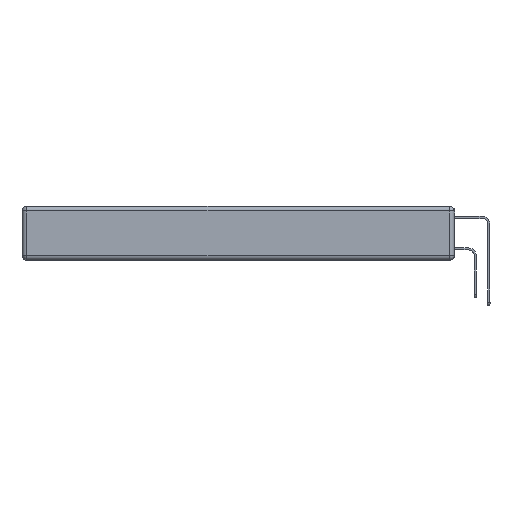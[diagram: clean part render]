
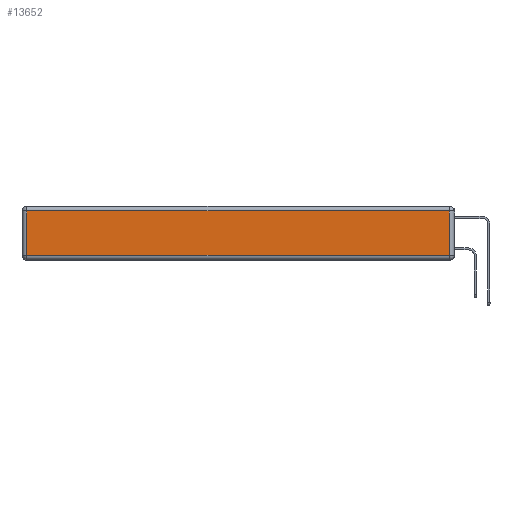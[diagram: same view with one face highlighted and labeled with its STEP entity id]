
A CAD part, left-side view. The second image highlights one B-rep face of the part: STEP entity #13652.
In plain terms, the highlighted planar face has unit normal (-1, 0, 0).
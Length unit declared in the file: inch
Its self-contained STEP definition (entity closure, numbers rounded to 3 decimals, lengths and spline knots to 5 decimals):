
#912 = CARTESIAN_POINT ( 'NONE',  ( 0., 0.03, -0.313 ) ) ;
#995 = DIRECTION ( 'NONE',  ( 0., 0., 1. ) ) ;
#1275 = LINE ( 'NONE', #16826, #14000 ) ;
#2342 = DIRECTION ( 'NONE',  ( 0., 0., 1. ) ) ;
#2383 = VERTEX_POINT ( 'NONE', #912 ) ;
#2860 = VERTEX_POINT ( 'NONE', #10020 ) ;
#2993 = VECTOR ( 'NONE', #8136, 39.37008 ) ;
#3424 = ORIENTED_EDGE ( 'NONE', *, *, #16909, .T. ) ;
#3539 = EDGE_CURVE ( 'NONE', #2860, #5676, #1275, .T. ) ;
#3596 = FACE_OUTER_BOUND ( 'NONE', #4056, .T. ) ;
#3638 = CARTESIAN_POINT ( 'NONE',  ( 0., 0.03, -0.343 ) ) ;
#4056 = EDGE_LOOP ( 'NONE', ( #3424, #6525, #5889, #4985 ) ) ;
#4985 = ORIENTED_EDGE ( 'NONE', *, *, #3539, .T. ) ;
#5272 = VECTOR ( 'NONE', #14107, 39.37008 ) ;
#5676 = VERTEX_POINT ( 'NONE', #12614 ) ;
#5889 = ORIENTED_EDGE ( 'NONE', *, *, #14051, .T. ) ;
#6525 = ORIENTED_EDGE ( 'NONE', *, *, #13401, .T. ) ;
#6547 = LINE ( 'NONE', #3638, #8463 ) ;
#8136 = DIRECTION ( 'NONE',  ( 0., -1., 0. ) ) ;
#8463 = VECTOR ( 'NONE', #2342, 39.37008 ) ;
#9367 = CARTESIAN_POINT ( 'NONE',  ( 0., 0., -0.313 ) ) ;
#9396 = AXIS2_PLACEMENT_3D ( 'NONE', #11524, #12802, #995 ) ;
#10020 = CARTESIAN_POINT ( 'NONE',  ( 0., 2.72, -0.03 ) ) ;
#10526 = DIRECTION ( 'NONE',  ( 0., 0., -1. ) ) ;
#11277 = VERTEX_POINT ( 'NONE', #15362 ) ;
#11524 = CARTESIAN_POINT ( 'NONE',  ( 0., 0., -0.343 ) ) ;
#12614 = CARTESIAN_POINT ( 'NONE',  ( 0., 2.72, -0.313 ) ) ;
#12802 = DIRECTION ( 'NONE',  ( -1., 0., 0. ) ) ;
#13401 = EDGE_CURVE ( 'NONE', #2383, #11277, #6547, .T. ) ;
#13489 = LINE ( 'NONE', #9367, #2993 ) ;
#13652 = ADVANCED_FACE ( 'NONE', ( #3596 ), #14032, .T. ) ;
#14000 = VECTOR ( 'NONE', #10526, 39.37008 ) ;
#14032 = PLANE ( 'NONE',  #9396 ) ;
#14051 = EDGE_CURVE ( 'NONE', #11277, #2860, #15219, .T. ) ;
#14107 = DIRECTION ( 'NONE',  ( 0., 1., 0. ) ) ;
#15219 = LINE ( 'NONE', #16780, #5272 ) ;
#15362 = CARTESIAN_POINT ( 'NONE',  ( 0., 0.03, -0.03 ) ) ;
#16780 = CARTESIAN_POINT ( 'NONE',  ( 0., 2.75, -0.03 ) ) ;
#16826 = CARTESIAN_POINT ( 'NONE',  ( 0., 2.72, -0.343 ) ) ;
#16909 = EDGE_CURVE ( 'NONE', #5676, #2383, #13489, .T. ) ;
